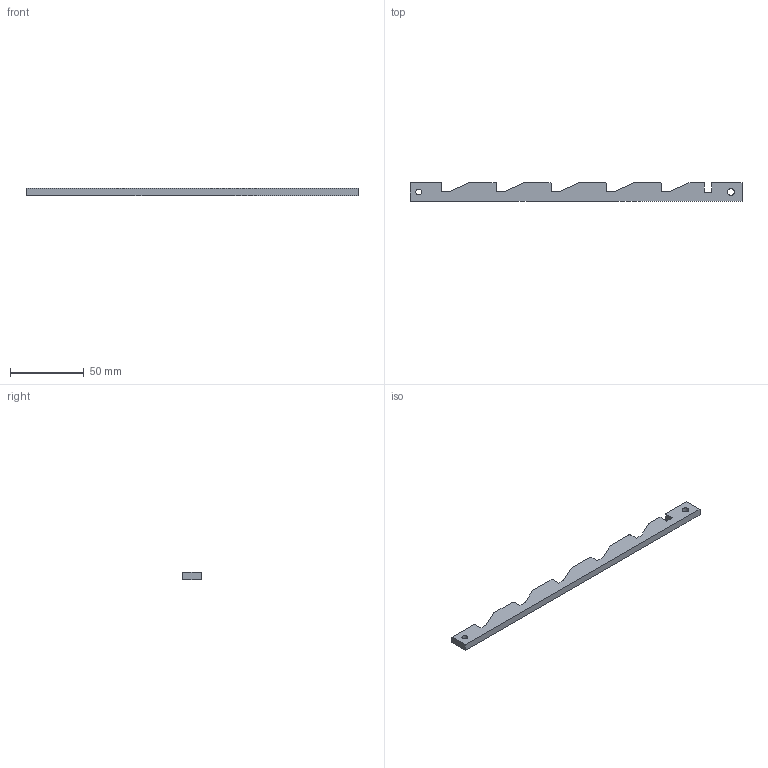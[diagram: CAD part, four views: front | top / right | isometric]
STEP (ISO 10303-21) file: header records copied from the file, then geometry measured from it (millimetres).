
FILE_DESCRIPTION(('FreeCAD Model'),'2;1');
FILE_NAME('Open CASCADE Shape Model','2024-04-24T10:01:29',('Author'),( ''),'Open CASCADE STEP processor 7.5','FreeCAD','Unknown');
FILE_SCHEMA(('AUTOMOTIVE_DESIGN { 1 0 10303 214 1 1 1 1 }'));
Length unit declared in the file: millimetre
Products named in the file (1): TelescopingBarRackCutArray
Bounding box: 225 x 12.7 x 4.76 mm (x, y, z)
Volume: 11535.1 mm3; surface area: 7472.5 mm2
Topology: 1 solids, 1 shells, 47 faces, 135 edges, 90 vertices
Faces by surface type: plane 30, cylinder 17
Full cylindrical faces by diameter (mm): 4 x1, 4.6 x1
Entity records: 3256 total; most frequent: CARTESIAN_POINT 615, DIRECTION 463, ORIENTED_EDGE 270, PCURVE 270, DEFINITIONAL_REPRESENTATION 270, LINE 265, VECTOR 265, EDGE_CURVE 135
